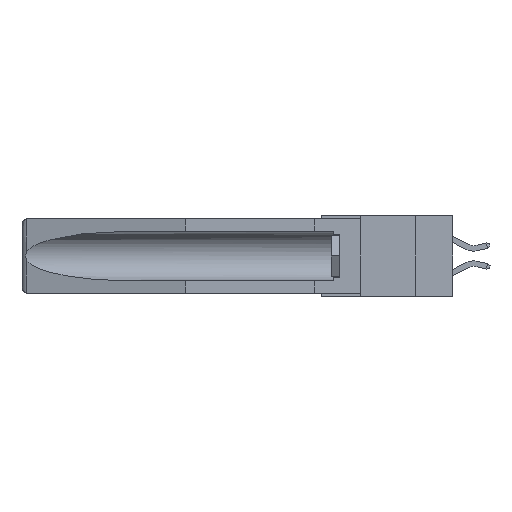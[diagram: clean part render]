
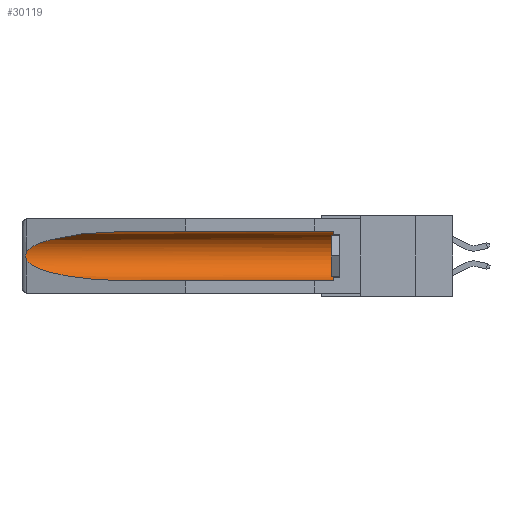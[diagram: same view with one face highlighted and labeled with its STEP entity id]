
A CAD part, left-side view. The second image highlights one B-rep face of the part: STEP entity #30119.
In plain terms, the highlighted cylindrical face has radius 2.857 mm (diameter 5.715 mm), a partial arc.
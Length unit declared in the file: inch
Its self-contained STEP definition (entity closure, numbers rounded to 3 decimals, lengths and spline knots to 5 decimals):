
#477 = VERTEX_POINT ( 'NONE', #24123 ) ;
#707 = VERTEX_POINT ( 'NONE', #1661 ) ;
#715 = DIRECTION ( 'NONE',  ( 0., 1., 0. ) ) ;
#838 = CARTESIAN_POINT ( 'NONE',  ( 0.21114, 1.30732, -0.284 ) ) ;
#971 = AXIS2_PLACEMENT_3D ( 'NONE', #8911, #16030, #3877 ) ;
#992 = ORIENTED_EDGE ( 'NONE', *, *, #23514, .T. ) ;
#1657 = CARTESIAN_POINT ( 'NONE',  ( 0.21114, 1.30732, -0.059 ) ) ;
#1661 = CARTESIAN_POINT ( 'NONE',  ( 0.26537, 1.52718, -0.19328 ) ) ;
#1761 = CARTESIAN_POINT ( 'NONE',  ( 0.25451, 1.48313, -0.09465 ) ) ;
#2133 =( BOUNDED_CURVE ( )  B_SPLINE_CURVE ( 3, ( #25560, #1657, #1761, #6308 ),
 .UNSPECIFIED., .F., .F. ) 
 B_SPLINE_CURVE_WITH_KNOTS ( ( 4, 4 ),
 ( 4.71239, 6.08839 ),
 .UNSPECIFIED. ) 
 CURVE ( )  GEOMETRIC_REPRESENTATION_ITEM ( )  RATIONAL_B_SPLINE_CURVE ( ( 1., 0.848, 0.848, 1. ) ) 
 REPRESENTATION_ITEM ( '' )  );
#2348 = CARTESIAN_POINT ( 'NONE',  ( 0.2675, 1.53308, -0.16763 ) ) ;
#2541 = VERTEX_POINT ( 'NONE', #18703 ) ;
#2710 = DIRECTION ( 'NONE',  ( 0., 1., 0. ) ) ;
#3121 = CARTESIAN_POINT ( 'NONE',  ( 0.155, -0.30754, -0.1715 ) ) ;
#3209 = CIRCLE ( 'NONE', #971, 0.1125 ) ;
#3877 = DIRECTION ( 'NONE',  ( 0., 0., 1. ) ) ;
#5453 = CARTESIAN_POINT ( 'NONE',  ( 0.155, -0.30754, -0.284 ) ) ;
#5982 = VERTEX_POINT ( 'NONE', #6479 ) ;
#6308 = CARTESIAN_POINT ( 'NONE',  ( 0.26537, 1.52718, -0.14972 ) ) ;
#6479 = CARTESIAN_POINT ( 'NONE',  ( 0.26537, 1.52718, -0.14972 ) ) ;
#6811 = CARTESIAN_POINT ( 'NONE',  ( 0.26597, 1.52961, -0.15275 ) ) ;
#6981 = ORIENTED_EDGE ( 'NONE', *, *, #16259, .T. ) ;
#7798 = CARTESIAN_POINT ( 'NONE',  ( 0.25451, 1.48313, -0.24835 ) ) ;
#8460 = ORIENTED_EDGE ( 'NONE', *, *, #13525, .T. ) ;
#8911 = CARTESIAN_POINT ( 'NONE',  ( 0.155, 0.126, -0.1715 ) ) ;
#9637 = CARTESIAN_POINT ( 'NONE',  ( 0.155, 0.126, -0.059 ) ) ;
#9815 =( BOUNDED_CURVE ( )  B_SPLINE_CURVE ( 3, ( #9925, #7798, #838, #12633 ),
 .UNSPECIFIED., .F., .F. ) 
 B_SPLINE_CURVE_WITH_KNOTS ( ( 4, 4 ),
 ( 0.1948, 1.5708 ),
 .UNSPECIFIED. ) 
 CURVE ( )  GEOMETRIC_REPRESENTATION_ITEM ( )  RATIONAL_B_SPLINE_CURVE ( ( 1., 0.848, 0.848, 1. ) ) 
 REPRESENTATION_ITEM ( '' )  );
#9925 = CARTESIAN_POINT ( 'NONE',  ( 0.26537, 1.52718, -0.19328 ) ) ;
#10519 = LINE ( 'NONE', #28087, #11254 ) ;
#10877 = ORIENTED_EDGE ( 'NONE', *, *, #30875, .T. ) ;
#10940 = EDGE_CURVE ( 'NONE', #477, #27364, #22093, .T. ) ;
#11254 = VECTOR ( 'NONE', #25797, 39.37008 ) ;
#11564 = ORIENTED_EDGE ( 'NONE', *, *, #10940, .F. ) ;
#12064 = CARTESIAN_POINT ( 'NONE',  ( 0.2673, 1.53269, -0.17917 ) ) ;
#12633 = CARTESIAN_POINT ( 'NONE',  ( 0.155, 1.07973, -0.284 ) ) ;
#13525 = EDGE_CURVE ( 'NONE', #707, #27364, #9815, .T. ) ;
#14068 = CARTESIAN_POINT ( 'NONE',  ( 0.26654, 1.53092, -0.15636 ) ) ;
#14170 = CARTESIAN_POINT ( 'NONE',  ( 0.26537, 1.52718, -0.19328 ) ) ;
#15703 = EDGE_LOOP ( 'NONE', ( #10877, #6981, #8460, #11564, #20151, #992 ) ) ;
#15759 = VECTOR ( 'NONE', #715, 39.37008 ) ;
#16030 = DIRECTION ( 'NONE',  ( 0., -1., 0. ) ) ;
#16259 = EDGE_CURVE ( 'NONE', #5982, #707, #30242, .T. ) ;
#16784 = CARTESIAN_POINT ( 'NONE',  ( 0.2673, 1.5327, -0.16383 ) ) ;
#18703 = CARTESIAN_POINT ( 'NONE',  ( 0.155, 1.07973, -0.059 ) ) ;
#20101 = EDGE_CURVE ( 'NONE', #477, #30041, #3209, .T. ) ;
#20151 = ORIENTED_EDGE ( 'NONE', *, *, #20101, .T. ) ;
#21262 = CARTESIAN_POINT ( 'NONE',  ( 0.26597, 1.5296, -0.19026 ) ) ;
#21356 = AXIS2_PLACEMENT_3D ( 'NONE', #3121, #2710, #29119 ) ;
#21468 = CARTESIAN_POINT ( 'NONE',  ( 0.26655, 1.53094, -0.18657 ) ) ;
#21769 = FACE_OUTER_BOUND ( 'NONE', #15703, .T. ) ;
#22093 = LINE ( 'NONE', #5453, #15759 ) ;
#23514 = EDGE_CURVE ( 'NONE', #30041, #2541, #10519, .T. ) ;
#24123 = CARTESIAN_POINT ( 'NONE',  ( 0.155, 0.126, -0.284 ) ) ;
#25560 = CARTESIAN_POINT ( 'NONE',  ( 0.155, 1.07973, -0.059 ) ) ;
#25797 = DIRECTION ( 'NONE',  ( 0., 1., 0. ) ) ;
#26383 = CARTESIAN_POINT ( 'NONE',  ( 0.2675, 1.53308, -0.17534 ) ) ;
#26623 = CYLINDRICAL_SURFACE ( 'NONE', #21356, 0.1125 ) ;
#27364 = VERTEX_POINT ( 'NONE', #27579 ) ;
#27579 = CARTESIAN_POINT ( 'NONE',  ( 0.155, 1.07973, -0.284 ) ) ;
#28087 = CARTESIAN_POINT ( 'NONE',  ( 0.155, -0.30754, -0.059 ) ) ;
#28350 = CARTESIAN_POINT ( 'NONE',  ( 0.26537, 1.52718, -0.14972 ) ) ;
#29119 = DIRECTION ( 'NONE',  ( 0., 0., 1. ) ) ;
#30041 = VERTEX_POINT ( 'NONE', #9637 ) ;
#30119 = ADVANCED_FACE ( 'NONE', ( #21769 ), #26623, .F. ) ;
#30242 = B_SPLINE_CURVE_WITH_KNOTS ( 'NONE', 3,
 ( #28350, #6811, #14068, #16784, #2348, #26383, #12064, #21468, #21262, #14170 ),
 .UNSPECIFIED., .F., .F.,
 ( 4, 2, 2, 2, 4 ),
 ( 0., 0.00029, 0.00058, 0.00087, 0.00117 ),
 .UNSPECIFIED. ) ;
#30875 = EDGE_CURVE ( 'NONE', #2541, #5982, #2133, .T. ) ;
